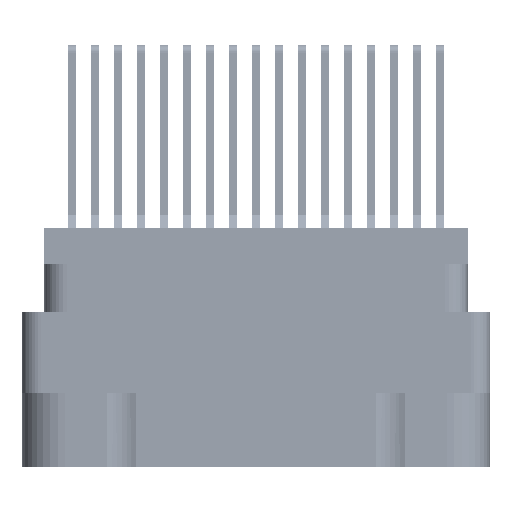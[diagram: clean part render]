
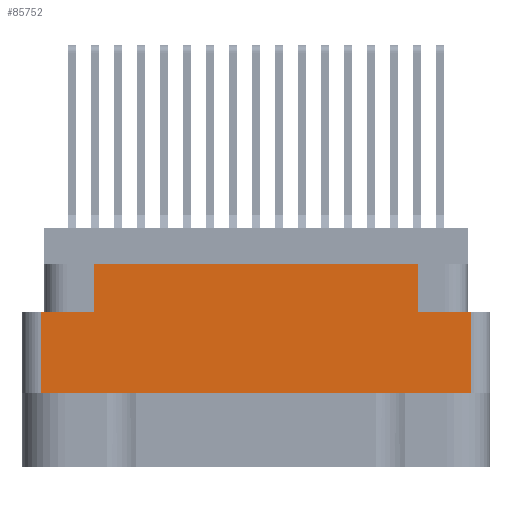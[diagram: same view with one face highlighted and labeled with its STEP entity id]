
A CAD part, left-side view. The second image highlights one B-rep face of the part: STEP entity #85752.
In plain terms, the highlighted planar face has unit normal (-1, 0, 0).
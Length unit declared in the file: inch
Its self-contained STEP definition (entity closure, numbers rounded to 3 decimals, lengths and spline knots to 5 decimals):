
#1224 = ORIENTED_EDGE ( 'NONE', *, *, #6988, .T. ) ;
#2466 = LINE ( 'NONE', #80559, #62381 ) ;
#2890 = CARTESIAN_POINT ( 'NONE',  ( -1.375, -0.7625, -0.78 ) ) ;
#3555 = LINE ( 'NONE', #7346, #36237 ) ;
#3798 = EDGE_CURVE ( 'NONE', #28461, #80050, #3555, .T. ) ;
#6988 = EDGE_CURVE ( 'NONE', #77517, #40830, #55796, .T. ) ;
#7346 = CARTESIAN_POINT ( 'NONE',  ( -1.375, 0.5285, -0.274 ) ) ;
#7922 = ORIENTED_EDGE ( 'NONE', *, *, #76144, .T. ) ;
#8537 = ORIENTED_EDGE ( 'NONE', *, *, #50278, .T. ) ;
#9271 = CARTESIAN_POINT ( 'NONE',  ( -1.375, 0.5285, -0.274 ) ) ;
#10341 = EDGE_CURVE ( 'NONE', #74111, #68224, #71436, .T. ) ;
#10961 = DIRECTION ( 'NONE',  ( 0., 0., -1. ) ) ;
#14736 = VERTEX_POINT ( 'NONE', #18672 ) ;
#14836 = VECTOR ( 'NONE', #85812, 39.37008 ) ;
#15426 = ORIENTED_EDGE ( 'NONE', *, *, #10341, .F. ) ;
#16373 = ORIENTED_EDGE ( 'NONE', *, *, #48673, .F. ) ;
#18546 = CARTESIAN_POINT ( 'NONE',  ( -1.375, -0.7005, -0.274 ) ) ;
#18672 = CARTESIAN_POINT ( 'NONE',  ( -1.375, -0.5285, -0.117 ) ) ;
#19509 = ORIENTED_EDGE ( 'NONE', *, *, #82960, .T. ) ;
#21132 = VECTOR ( 'NONE', #40892, 39.37008 ) ;
#22380 = DIRECTION ( 'NONE',  ( -1., 0., 0. ) ) ;
#22725 = CARTESIAN_POINT ( 'NONE',  ( -1.375, 0.7005, -0.274 ) ) ;
#23635 = DIRECTION ( 'NONE',  ( 0., -1., 0. ) ) ;
#24407 = CARTESIAN_POINT ( 'NONE',  ( -1.375, 0.7005, -0.54 ) ) ;
#28461 = VERTEX_POINT ( 'NONE', #9271 ) ;
#30885 = VECTOR ( 'NONE', #10961, 39.37008 ) ;
#33761 = ORIENTED_EDGE ( 'NONE', *, *, #86271, .F. ) ;
#35610 = PLANE ( 'NONE',  #47763 ) ;
#36237 = VECTOR ( 'NONE', #61105, 39.37008 ) ;
#39133 = VERTEX_POINT ( 'NONE', #22725 ) ;
#39351 = CARTESIAN_POINT ( 'NONE',  ( -1.375, -0.7005, -0.78 ) ) ;
#40830 = VERTEX_POINT ( 'NONE', #45949 ) ;
#40892 = DIRECTION ( 'NONE',  ( 0., -1., 0. ) ) ;
#42379 = DIRECTION ( 'NONE',  ( 0., -1., 0. ) ) ;
#42912 = LINE ( 'NONE', #44264, #56479 ) ;
#42990 = VECTOR ( 'NONE', #42379, 39.37008 ) ;
#44264 = CARTESIAN_POINT ( 'NONE',  ( -1.375, 0.7625, -0.117 ) ) ;
#45949 = CARTESIAN_POINT ( 'NONE',  ( -1.375, -0.7005, -0.54 ) ) ;
#46759 = ORIENTED_EDGE ( 'NONE', *, *, #3798, .F. ) ;
#47763 = AXIS2_PLACEMENT_3D ( 'NONE', #2890, #22380, #63119 ) ;
#48673 = EDGE_CURVE ( 'NONE', #39133, #28461, #74289, .T. ) ;
#50278 = EDGE_CURVE ( 'NONE', #74111, #14736, #2466, .T. ) ;
#53738 = CARTESIAN_POINT ( 'NONE',  ( -1.375, -0.5285, -0.274 ) ) ;
#55796 = LINE ( 'NONE', #59151, #76667 ) ;
#56479 = VECTOR ( 'NONE', #23635, 39.37008 ) ;
#57576 = CARTESIAN_POINT ( 'NONE',  ( -1.375, 0.5285, -0.117 ) ) ;
#59134 = EDGE_LOOP ( 'NONE', ( #16373, #19509, #1224, #7922, #15426, #8537, #33761, #46759 ) ) ;
#59151 = CARTESIAN_POINT ( 'NONE',  ( -1.375, 0., -0.54 ) ) ;
#60658 = DIRECTION ( 'NONE',  ( 0., 0., 1. ) ) ;
#61105 = DIRECTION ( 'NONE',  ( 0., 0., 1. ) ) ;
#62381 = VECTOR ( 'NONE', #60658, 39.37008 ) ;
#63119 = DIRECTION ( 'NONE',  ( 0., 0., 1. ) ) ;
#64391 = CARTESIAN_POINT ( 'NONE',  ( -1.375, 0.7005, -0.78 ) ) ;
#68224 = VERTEX_POINT ( 'NONE', #18546 ) ;
#68907 = CARTESIAN_POINT ( 'NONE',  ( -1.375, 0., -0.274 ) ) ;
#71436 = LINE ( 'NONE', #68907, #21132 ) ;
#72617 = LINE ( 'NONE', #39351, #14836 ) ;
#73711 = DIRECTION ( 'NONE',  ( 0., -1., 0. ) ) ;
#74111 = VERTEX_POINT ( 'NONE', #53738 ) ;
#74289 = LINE ( 'NONE', #81475, #42990 ) ;
#76144 = EDGE_CURVE ( 'NONE', #40830, #68224, #72617, .T. ) ;
#76667 = VECTOR ( 'NONE', #73711, 39.37008 ) ;
#77517 = VERTEX_POINT ( 'NONE', #24407 ) ;
#78538 = FACE_OUTER_BOUND ( 'NONE', #59134, .T. ) ;
#80050 = VERTEX_POINT ( 'NONE', #57576 ) ;
#80559 = CARTESIAN_POINT ( 'NONE',  ( -1.375, -0.5285, -0.274 ) ) ;
#81475 = CARTESIAN_POINT ( 'NONE',  ( -1.375, 0., -0.274 ) ) ;
#82960 = EDGE_CURVE ( 'NONE', #39133, #77517, #86372, .T. ) ;
#85752 = ADVANCED_FACE ( 'NONE', ( #78538 ), #35610, .T. ) ;
#85812 = DIRECTION ( 'NONE',  ( 0., 0., 1. ) ) ;
#86271 = EDGE_CURVE ( 'NONE', #80050, #14736, #42912, .T. ) ;
#86372 = LINE ( 'NONE', #64391, #30885 ) ;
